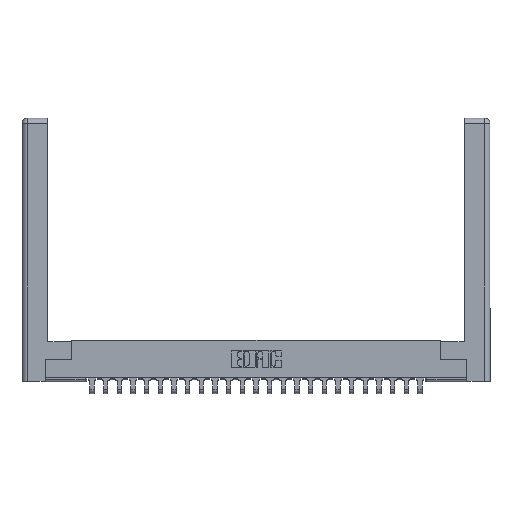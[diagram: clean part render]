
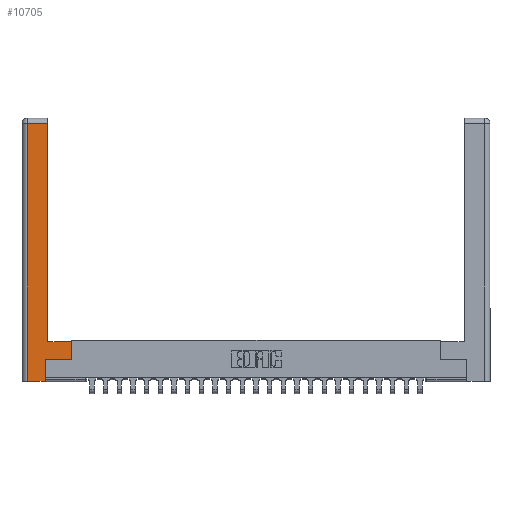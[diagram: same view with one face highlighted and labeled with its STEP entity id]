
A CAD part, top view. The second image highlights one B-rep face of the part: STEP entity #10705.
In plain terms, the highlighted planar face has unit normal (0, 0, 1).
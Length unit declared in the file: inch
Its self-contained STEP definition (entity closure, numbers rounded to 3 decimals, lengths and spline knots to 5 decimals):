
#162 = CARTESIAN_POINT ( 'NONE',  ( 0.0615, 2.94, 0. ) ) ;
#222 = CARTESIAN_POINT ( 'NONE',  ( 0.565, 0.45, 0. ) ) ;
#263 = DIRECTION ( 'NONE',  ( 0., 1., 0. ) ) ;
#316 = CARTESIAN_POINT ( 'NONE',  ( 0.295, 0.45, 0. ) ) ;
#345 = LINE ( 'NONE', #17793, #3789 ) ;
#1778 = CARTESIAN_POINT ( 'NONE',  ( 0.0615, 0., 0. ) ) ;
#1854 = EDGE_CURVE ( 'NONE', #21397, #14021, #345, .T. ) ;
#2293 = CARTESIAN_POINT ( 'NONE',  ( 0.265, 0., 0. ) ) ;
#3789 = VECTOR ( 'NONE', #13793, 39.37008 ) ;
#3914 = PLANE ( 'NONE',  #7545 ) ;
#4061 = LINE ( 'NONE', #1778, #9413 ) ;
#5244 = VERTEX_POINT ( 'NONE', #24063 ) ;
#5378 = VERTEX_POINT ( 'NONE', #162 ) ;
#5962 = CARTESIAN_POINT ( 'NONE',  ( 0., 0., 0. ) ) ;
#6172 = CARTESIAN_POINT ( 'NONE',  ( 0.295, 3., 0. ) ) ;
#6531 = DIRECTION ( 'NONE',  ( 1., 0., 0. ) ) ;
#7545 = AXIS2_PLACEMENT_3D ( 'NONE', #5962, #11886, #13915 ) ;
#8034 = CARTESIAN_POINT ( 'NONE',  ( 0.565, 0.245, 0. ) ) ;
#8265 = VERTEX_POINT ( 'NONE', #8034 ) ;
#8293 = VECTOR ( 'NONE', #6531, 39.37008 ) ;
#9337 = CARTESIAN_POINT ( 'NONE',  ( 0.295, 0.45, 0. ) ) ;
#9413 = VECTOR ( 'NONE', #26253, 39.37008 ) ;
#10320 = VERTEX_POINT ( 'NONE', #16929 ) ;
#10582 = ORIENTED_EDGE ( 'NONE', *, *, #22214, .T. ) ;
#10591 = CARTESIAN_POINT ( 'NONE',  ( 0.0615, 2.94, 0. ) ) ;
#10705 = ADVANCED_FACE ( 'NONE', ( #20007 ), #3914, .F. ) ;
#10869 = CARTESIAN_POINT ( 'NONE',  ( 0.0615, 0., 0. ) ) ;
#11564 = EDGE_CURVE ( 'NONE', #8265, #10320, #24720, .T. ) ;
#11686 = ORIENTED_EDGE ( 'NONE', *, *, #13224, .T. ) ;
#11886 = DIRECTION ( 'NONE',  ( 0., 0., -1. ) ) ;
#12308 = EDGE_LOOP ( 'NONE', ( #13063, #11686, #16953, #13626, #23606, #10582, #13403, #17272 ) ) ;
#12788 = LINE ( 'NONE', #6172, #23284 ) ;
#13063 = ORIENTED_EDGE ( 'NONE', *, *, #14348, .T. ) ;
#13224 = EDGE_CURVE ( 'NONE', #5244, #5378, #23997, .T. ) ;
#13403 = ORIENTED_EDGE ( 'NONE', *, *, #11564, .T. ) ;
#13626 = ORIENTED_EDGE ( 'NONE', *, *, #25586, .T. ) ;
#13653 = LINE ( 'NONE', #2293, #8293 ) ;
#13793 = DIRECTION ( 'NONE',  ( 0., 1., 0. ) ) ;
#13915 = DIRECTION ( 'NONE',  ( -1., 0., 0. ) ) ;
#14021 = VERTEX_POINT ( 'NONE', #20408 ) ;
#14125 = LINE ( 'NONE', #316, #18885 ) ;
#14318 = DIRECTION ( 'NONE',  ( 1., 0., 0. ) ) ;
#14348 = EDGE_CURVE ( 'NONE', #22028, #5244, #12788, .T. ) ;
#14477 = LINE ( 'NONE', #16350, #22741 ) ;
#16350 = CARTESIAN_POINT ( 'NONE',  ( 0.565, 0.245, 0. ) ) ;
#16397 = DIRECTION ( 'NONE',  ( 0., 1., 0. ) ) ;
#16929 = CARTESIAN_POINT ( 'NONE',  ( 0.565, 0.45, 0. ) ) ;
#16953 = ORIENTED_EDGE ( 'NONE', *, *, #19865, .T. ) ;
#17272 = ORIENTED_EDGE ( 'NONE', *, *, #22846, .T. ) ;
#17696 = VERTEX_POINT ( 'NONE', #10869 ) ;
#17793 = CARTESIAN_POINT ( 'NONE',  ( 0.265, 0.245, 0. ) ) ;
#18550 = DIRECTION ( 'NONE',  ( -1., 0., 0. ) ) ;
#18885 = VECTOR ( 'NONE', #18550, 39.37008 ) ;
#19296 = CARTESIAN_POINT ( 'NONE',  ( 0.265, 0., 0. ) ) ;
#19865 = EDGE_CURVE ( 'NONE', #5378, #17696, #4061, .T. ) ;
#20007 = FACE_OUTER_BOUND ( 'NONE', #12308, .T. ) ;
#20408 = CARTESIAN_POINT ( 'NONE',  ( 0.265, 0.245, 0. ) ) ;
#20642 = DIRECTION ( 'NONE',  ( -1., 0., 0. ) ) ;
#21397 = VERTEX_POINT ( 'NONE', #19296 ) ;
#21447 = VECTOR ( 'NONE', #20642, 39.37008 ) ;
#22028 = VERTEX_POINT ( 'NONE', #9337 ) ;
#22214 = EDGE_CURVE ( 'NONE', #14021, #8265, #14477, .T. ) ;
#22741 = VECTOR ( 'NONE', #14318, 39.37008 ) ;
#22846 = EDGE_CURVE ( 'NONE', #10320, #22028, #14125, .T. ) ;
#23101 = VECTOR ( 'NONE', #16397, 39.37008 ) ;
#23284 = VECTOR ( 'NONE', #263, 39.37008 ) ;
#23606 = ORIENTED_EDGE ( 'NONE', *, *, #1854, .T. ) ;
#23997 = LINE ( 'NONE', #10591, #21447 ) ;
#24063 = CARTESIAN_POINT ( 'NONE',  ( 0.295, 2.94, 0. ) ) ;
#24720 = LINE ( 'NONE', #222, #23101 ) ;
#25586 = EDGE_CURVE ( 'NONE', #17696, #21397, #13653, .T. ) ;
#26253 = DIRECTION ( 'NONE',  ( 0., -1., 0. ) ) ;
